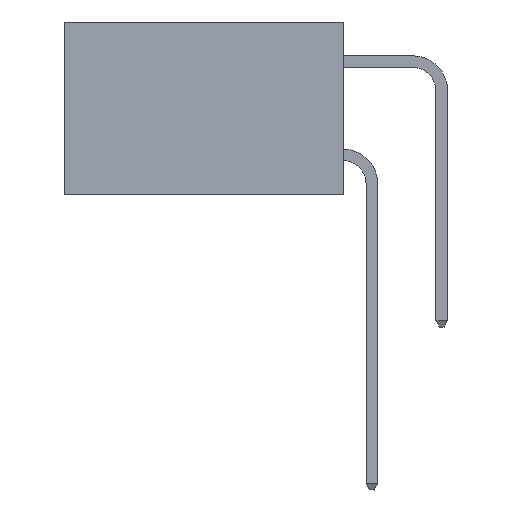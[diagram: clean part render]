
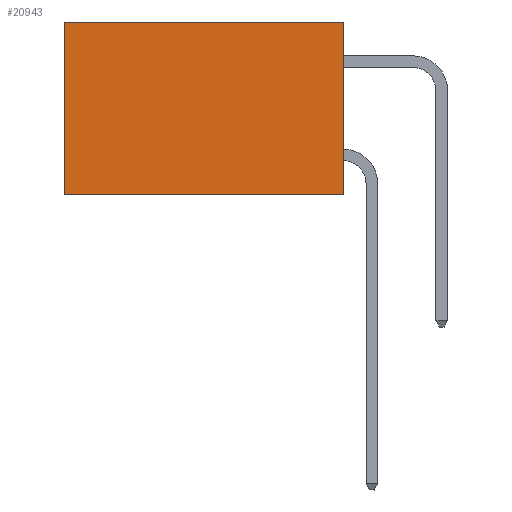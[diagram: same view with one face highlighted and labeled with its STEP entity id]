
A CAD part, left-side view. The second image highlights one B-rep face of the part: STEP entity #20943.
In plain terms, the highlighted planar face has unit normal (-1, 0, 0).
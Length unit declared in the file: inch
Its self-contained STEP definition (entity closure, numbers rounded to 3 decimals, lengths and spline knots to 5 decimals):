
#291 = ORIENTED_EDGE ( 'NONE', *, *, #9553, .T. ) ;
#366 = VECTOR ( 'NONE', #20267, 39.37008 ) ;
#915 = CARTESIAN_POINT ( 'NONE',  ( 0.2615, 0.6, -0.37 ) ) ;
#1028 = FACE_OUTER_BOUND ( 'NONE', #12322, .T. ) ;
#1157 = VECTOR ( 'NONE', #18922, 39.37008 ) ;
#3254 = LINE ( 'NONE', #5022, #1157 ) ;
#4216 = VERTEX_POINT ( 'NONE', #22043 ) ;
#4681 = CARTESIAN_POINT ( 'NONE',  ( 0.2615, 0., -0.37 ) ) ;
#5022 = CARTESIAN_POINT ( 'NONE',  ( 0.2615, 0., 0. ) ) ;
#5644 = ORIENTED_EDGE ( 'NONE', *, *, #13494, .F. ) ;
#5697 = LINE ( 'NONE', #21020, #11618 ) ;
#5796 = CARTESIAN_POINT ( 'NONE',  ( 0.2615, 0., -0.37 ) ) ;
#6096 = EDGE_CURVE ( 'NONE', #6870, #4216, #18246, .T. ) ;
#6870 = VERTEX_POINT ( 'NONE', #23865 ) ;
#8720 = DIRECTION ( 'NONE',  ( 1., 0., 0. ) ) ;
#9553 = EDGE_CURVE ( 'NONE', #10266, #6870, #3254, .T. ) ;
#9812 = VECTOR ( 'NONE', #24901, 39.37008 ) ;
#10266 = VERTEX_POINT ( 'NONE', #21911 ) ;
#11503 = DIRECTION ( 'NONE',  ( 0., 0., -1. ) ) ;
#11618 = VECTOR ( 'NONE', #11503, 39.37008 ) ;
#12201 = ORIENTED_EDGE ( 'NONE', *, *, #21447, .F. ) ;
#12322 = EDGE_LOOP ( 'NONE', ( #14405, #12201, #5644, #291 ) ) ;
#13494 = EDGE_CURVE ( 'NONE', #10266, #23705, #5697, .T. ) ;
#14405 = ORIENTED_EDGE ( 'NONE', *, *, #6096, .T. ) ;
#16465 = DIRECTION ( 'NONE',  ( 0., 0., -1. ) ) ;
#16596 = PLANE ( 'NONE',  #24350 ) ;
#18246 = LINE ( 'NONE', #915, #366 ) ;
#18922 = DIRECTION ( 'NONE',  ( 0., 1., 0. ) ) ;
#20267 = DIRECTION ( 'NONE',  ( 0., 0., -1. ) ) ;
#20943 = ADVANCED_FACE ( 'NONE', ( #1028 ), #16596, .F. ) ;
#20997 = LINE ( 'NONE', #5796, #9812 ) ;
#21020 = CARTESIAN_POINT ( 'NONE',  ( 0.2615, 0., -0.37 ) ) ;
#21183 = CARTESIAN_POINT ( 'NONE',  ( 0.2615, 0., -0.37 ) ) ;
#21447 = EDGE_CURVE ( 'NONE', #23705, #4216, #20997, .T. ) ;
#21911 = CARTESIAN_POINT ( 'NONE',  ( 0.2615, 0., 0. ) ) ;
#22043 = CARTESIAN_POINT ( 'NONE',  ( 0.2615, 0.6, -0.37 ) ) ;
#23705 = VERTEX_POINT ( 'NONE', #21183 ) ;
#23865 = CARTESIAN_POINT ( 'NONE',  ( 0.2615, 0.6, 0. ) ) ;
#24350 = AXIS2_PLACEMENT_3D ( 'NONE', #4681, #8720, #16465 ) ;
#24901 = DIRECTION ( 'NONE',  ( 0., 1., 0. ) ) ;
